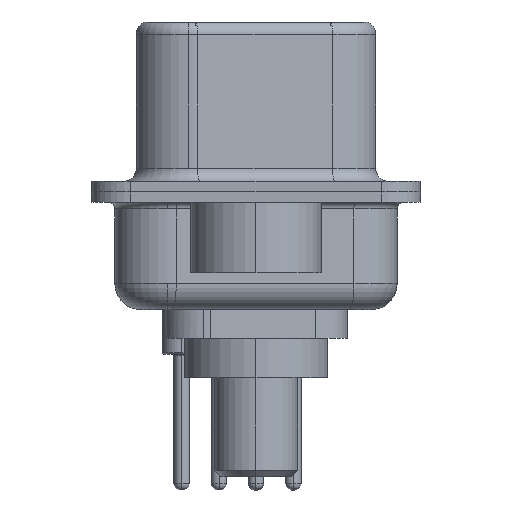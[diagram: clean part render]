
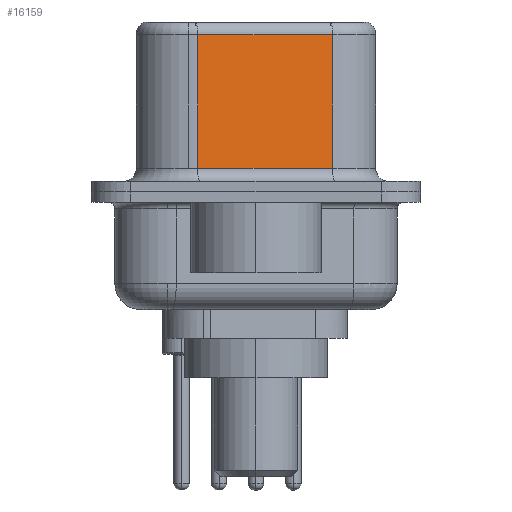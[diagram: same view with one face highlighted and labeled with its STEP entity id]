
A CAD part, left-side view. The second image highlights one B-rep face of the part: STEP entity #16159.
In plain terms, the highlighted planar face has unit normal (-0.985, -0.174, 0).
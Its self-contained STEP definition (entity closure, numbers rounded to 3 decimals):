
#393 = ORIENTED_EDGE ( 'NONE', *, *, #12618, .T. ) ;
#776 = EDGE_CURVE ( 'NONE', #13240, #6305, #19747, .T. ) ;
#1263 = DIRECTION ( 'NONE',  ( 0.985, 0.174, 0. ) ) ;
#1304 = CARTESIAN_POINT ( 'NONE',  ( 3.67, 2.233, 6.52 ) ) ;
#1970 = LINE ( 'NONE', #12181, #20429 ) ;
#3684 = VECTOR ( 'NONE', #7900, 1000. ) ;
#4770 = LINE ( 'NONE', #7966, #3684 ) ;
#4772 = DIRECTION ( 'NONE',  ( 0., 0., -1. ) ) ;
#4867 = EDGE_CURVE ( 'NONE', #10226, #19142, #4770, .T. ) ;
#6041 = CARTESIAN_POINT ( 'NONE',  ( 4.58, -2.927, 6.02 ) ) ;
#6305 = VERTEX_POINT ( 'NONE', #6791 ) ;
#6791 = CARTESIAN_POINT ( 'NONE',  ( 3.67, 2.233, 6.02 ) ) ;
#6815 = CARTESIAN_POINT ( 'NONE',  ( 4.58, -2.927, 6.02 ) ) ;
#7464 = VECTOR ( 'NONE', #4772, 1000. ) ;
#7639 = EDGE_CURVE ( 'NONE', #13240, #19142, #1970, .T. ) ;
#7832 = DIRECTION ( 'NONE',  ( -0.174, 0.985, 0. ) ) ;
#7900 = DIRECTION ( 'NONE',  ( 0.174, -0.985, 0. ) ) ;
#7966 = CARTESIAN_POINT ( 'NONE',  ( 4.58, -2.927, 0.9 ) ) ;
#9937 = PLANE ( 'NONE',  #12529 ) ;
#10226 = VERTEX_POINT ( 'NONE', #16386 ) ;
#11441 = FACE_OUTER_BOUND ( 'NONE', #20287, .T. ) ;
#12181 = CARTESIAN_POINT ( 'NONE',  ( 4.58, -2.927, 6.52 ) ) ;
#12529 = AXIS2_PLACEMENT_3D ( 'NONE', #22101, #1263, #13418 ) ;
#12618 = EDGE_CURVE ( 'NONE', #6305, #10226, #21331, .T. ) ;
#13240 = VERTEX_POINT ( 'NONE', #6815 ) ;
#13418 = DIRECTION ( 'NONE',  ( -0.174, 0.985, 0. ) ) ;
#14440 = CARTESIAN_POINT ( 'NONE',  ( 4.58, -2.927, 0.9 ) ) ;
#14619 = VECTOR ( 'NONE', #7832, 1000. ) ;
#15561 = ORIENTED_EDGE ( 'NONE', *, *, #776, .T. ) ;
#15757 = ORIENTED_EDGE ( 'NONE', *, *, #7639, .F. ) ;
#16159 = ADVANCED_FACE ( 'NONE', ( #11441 ), #9937, .F. ) ;
#16386 = CARTESIAN_POINT ( 'NONE',  ( 3.67, 2.233, 0.9 ) ) ;
#17409 = ORIENTED_EDGE ( 'NONE', *, *, #4867, .T. ) ;
#19142 = VERTEX_POINT ( 'NONE', #14440 ) ;
#19747 = LINE ( 'NONE', #6041, #14619 ) ;
#20287 = EDGE_LOOP ( 'NONE', ( #15757, #15561, #393, #17409 ) ) ;
#20429 = VECTOR ( 'NONE', #22602, 1000. ) ;
#21331 = LINE ( 'NONE', #1304, #7464 ) ;
#22101 = CARTESIAN_POINT ( 'NONE',  ( 4.58, -2.927, 6.52 ) ) ;
#22602 = DIRECTION ( 'NONE',  ( 0., 0., -1. ) ) ;
